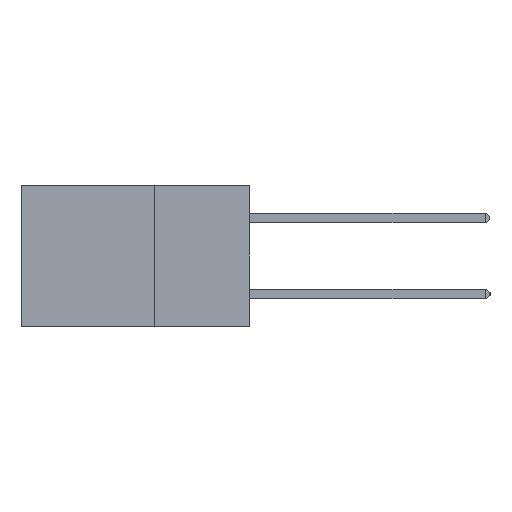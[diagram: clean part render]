
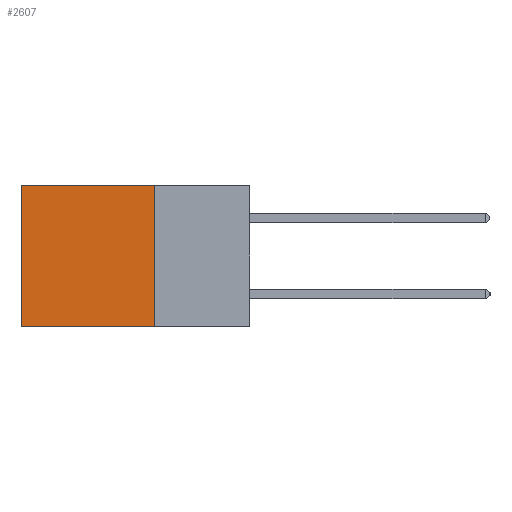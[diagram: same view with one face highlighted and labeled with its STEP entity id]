
A CAD part, left-side view. The second image highlights one B-rep face of the part: STEP entity #2607.
In plain terms, the highlighted planar face has unit normal (-1, 0, 0).
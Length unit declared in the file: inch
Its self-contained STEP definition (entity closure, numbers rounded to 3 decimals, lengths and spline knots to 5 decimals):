
#431 = EDGE_LOOP ( 'NONE', ( #4143, #15346, #11946, #20469 ) ) ;
#1310 = CARTESIAN_POINT ( 'NONE',  ( 0.2875, 0.25, 0. ) ) ;
#1762 = DIRECTION ( 'NONE',  ( 1., 0., 0. ) ) ;
#1954 = VECTOR ( 'NONE', #14431, 39.37008 ) ;
#2124 = AXIS2_PLACEMENT_3D ( 'NONE', #8875, #1762, #13827 ) ;
#2607 = ADVANCED_FACE ( 'NONE', ( #16124 ), #12217, .F. ) ;
#3064 = LINE ( 'NONE', #10791, #19902 ) ;
#3343 = EDGE_CURVE ( 'NONE', #15700, #20254, #15563, .T. ) ;
#4143 = ORIENTED_EDGE ( 'NONE', *, *, #21424, .T. ) ;
#4873 = LINE ( 'NONE', #14933, #17137 ) ;
#5299 = VERTEX_POINT ( 'NONE', #15685 ) ;
#8261 = VERTEX_POINT ( 'NONE', #10852 ) ;
#8875 = CARTESIAN_POINT ( 'NONE',  ( 0.2875, 0.25, 0. ) ) ;
#9571 = CARTESIAN_POINT ( 'NONE',  ( 0.2875, 0.6, 0. ) ) ;
#10791 = CARTESIAN_POINT ( 'NONE',  ( 0.2875, 0.25, 0. ) ) ;
#10852 = CARTESIAN_POINT ( 'NONE',  ( 0.2875, 0.6, -0.37 ) ) ;
#11801 = CARTESIAN_POINT ( 'NONE',  ( 0.2875, 0.25, -0.37 ) ) ;
#11946 = ORIENTED_EDGE ( 'NONE', *, *, #3343, .F. ) ;
#12217 = PLANE ( 'NONE',  #2124 ) ;
#12823 = CARTESIAN_POINT ( 'NONE',  ( 0.2875, 0.25, 0. ) ) ;
#12941 = EDGE_CURVE ( 'NONE', #20254, #8261, #4873, .T. ) ;
#13827 = DIRECTION ( 'NONE',  ( 0., 0., -1. ) ) ;
#14027 = DIRECTION ( 'NONE',  ( 0., 1., 0. ) ) ;
#14431 = DIRECTION ( 'NONE',  ( 0., 0., -1. ) ) ;
#14933 = CARTESIAN_POINT ( 'NONE',  ( 0.2875, 0.25, -0.37 ) ) ;
#15222 = EDGE_CURVE ( 'NONE', #15700, #5299, #3064, .T. ) ;
#15346 = ORIENTED_EDGE ( 'NONE', *, *, #12941, .F. ) ;
#15523 = VECTOR ( 'NONE', #19337, 39.37008 ) ;
#15563 = LINE ( 'NONE', #12823, #1954 ) ;
#15685 = CARTESIAN_POINT ( 'NONE',  ( 0.2875, 0.6, 0. ) ) ;
#15700 = VERTEX_POINT ( 'NONE', #1310 ) ;
#16037 = LINE ( 'NONE', #9571, #15523 ) ;
#16124 = FACE_OUTER_BOUND ( 'NONE', #431, .T. ) ;
#17137 = VECTOR ( 'NONE', #21427, 39.37008 ) ;
#19337 = DIRECTION ( 'NONE',  ( 0., 0., -1. ) ) ;
#19902 = VECTOR ( 'NONE', #14027, 39.37008 ) ;
#20254 = VERTEX_POINT ( 'NONE', #11801 ) ;
#20469 = ORIENTED_EDGE ( 'NONE', *, *, #15222, .T. ) ;
#21424 = EDGE_CURVE ( 'NONE', #5299, #8261, #16037, .T. ) ;
#21427 = DIRECTION ( 'NONE',  ( 0., 1., 0. ) ) ;
